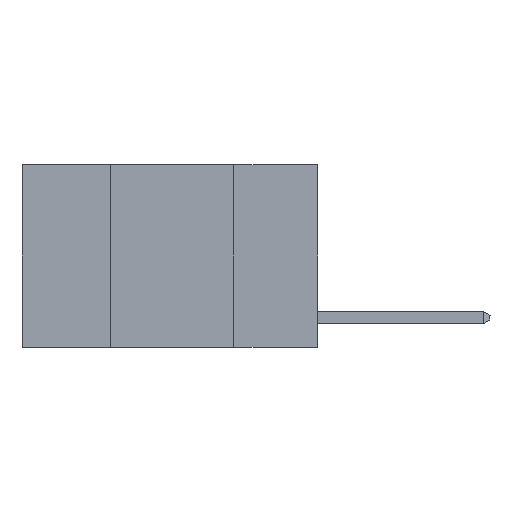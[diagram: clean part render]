
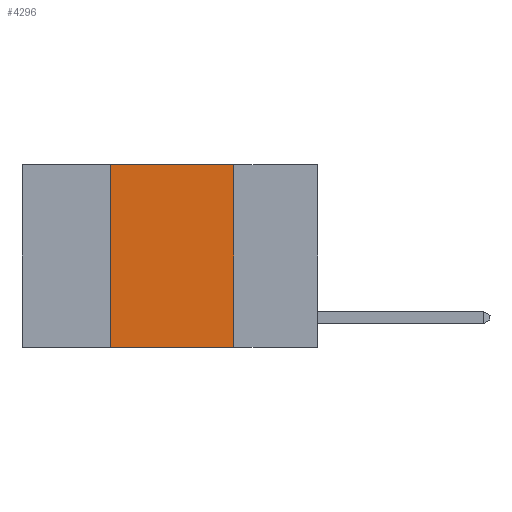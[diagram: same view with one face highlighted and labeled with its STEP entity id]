
A CAD part, left-side view. The second image highlights one B-rep face of the part: STEP entity #4296.
In plain terms, the highlighted planar face has unit normal (-1, 0, 0).
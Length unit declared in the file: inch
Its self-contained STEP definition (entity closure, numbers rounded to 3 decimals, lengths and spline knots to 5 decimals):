
#133 = VECTOR ( 'NONE', #3641, 39.37008 ) ;
#184 = EDGE_LOOP ( 'NONE', ( #5871, #4070, #5665, #3859 ) ) ;
#452 = DIRECTION ( 'NONE',  ( 1., 0., 0. ) ) ;
#944 = DIRECTION ( 'NONE',  ( 0., 0., -1. ) ) ;
#1072 = CARTESIAN_POINT ( 'NONE',  ( 0., 0.6, 0. ) ) ;
#1268 = DIRECTION ( 'NONE',  ( 0., 0., -1. ) ) ;
#1622 = CARTESIAN_POINT ( 'NONE',  ( 0., 0.6, -0.37 ) ) ;
#1864 = CARTESIAN_POINT ( 'NONE',  ( 0., 0.6, 0. ) ) ;
#1955 = DIRECTION ( 'NONE',  ( 0., 0., 1. ) ) ;
#2282 = LINE ( 'NONE', #4159, #7649 ) ;
#2735 = VERTEX_POINT ( 'NONE', #7073 ) ;
#2962 = AXIS2_PLACEMENT_3D ( 'NONE', #1864, #452, #1268 ) ;
#3641 = DIRECTION ( 'NONE',  ( 0., -1., 0. ) ) ;
#3859 = ORIENTED_EDGE ( 'NONE', *, *, #5804, .T. ) ;
#4070 = ORIENTED_EDGE ( 'NONE', *, *, #5868, .F. ) ;
#4159 = CARTESIAN_POINT ( 'NONE',  ( 0., 0.17, 0. ) ) ;
#4296 = ADVANCED_FACE ( 'NONE', ( #4624 ), #7916, .F. ) ;
#4464 = VECTOR ( 'NONE', #1955, 39.37008 ) ;
#4624 = FACE_OUTER_BOUND ( 'NONE', #184, .T. ) ;
#4654 = EDGE_CURVE ( 'NONE', #2735, #6254, #2282, .T. ) ;
#5127 = EDGE_CURVE ( 'NONE', #7041, #7279, #8008, .T. ) ;
#5630 = VECTOR ( 'NONE', #6360, 39.37008 ) ;
#5665 = ORIENTED_EDGE ( 'NONE', *, *, #5127, .F. ) ;
#5804 = EDGE_CURVE ( 'NONE', #7041, #6254, #8575, .T. ) ;
#5868 = EDGE_CURVE ( 'NONE', #7279, #2735, #7945, .T. ) ;
#5871 = ORIENTED_EDGE ( 'NONE', *, *, #4654, .F. ) ;
#6245 = CARTESIAN_POINT ( 'NONE',  ( 0., 0.42, 0. ) ) ;
#6254 = VERTEX_POINT ( 'NONE', #7531 ) ;
#6360 = DIRECTION ( 'NONE',  ( 0., -1., 0. ) ) ;
#6849 = CARTESIAN_POINT ( 'NONE',  ( 0., 0.42, -0.37 ) ) ;
#7041 = VERTEX_POINT ( 'NONE', #6849 ) ;
#7073 = CARTESIAN_POINT ( 'NONE',  ( 0., 0.17, 0. ) ) ;
#7279 = VERTEX_POINT ( 'NONE', #6245 ) ;
#7531 = CARTESIAN_POINT ( 'NONE',  ( 0., 0.17, -0.37 ) ) ;
#7649 = VECTOR ( 'NONE', #944, 39.37008 ) ;
#7916 = PLANE ( 'NONE',  #2962 ) ;
#7945 = LINE ( 'NONE', #1072, #5630 ) ;
#8008 = LINE ( 'NONE', #8628, #4464 ) ;
#8575 = LINE ( 'NONE', #1622, #133 ) ;
#8628 = CARTESIAN_POINT ( 'NONE',  ( 0., 0.42, 0. ) ) ;
